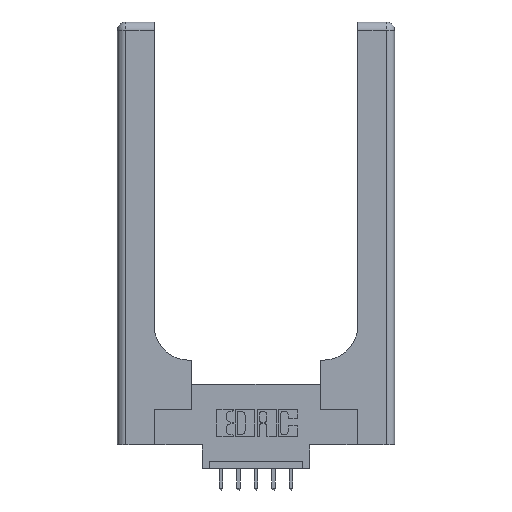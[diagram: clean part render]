
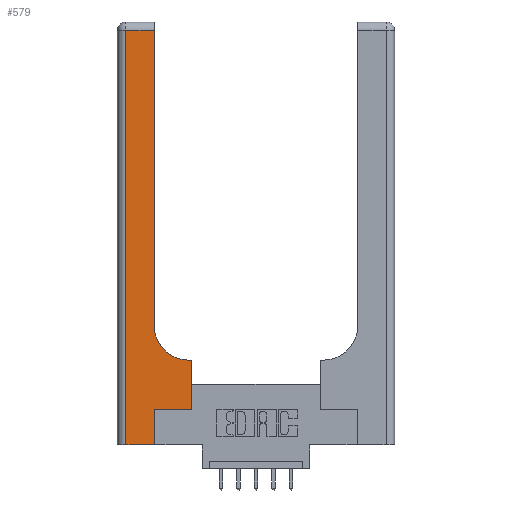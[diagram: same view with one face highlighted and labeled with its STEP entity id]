
A CAD part, top view. The second image highlights one B-rep face of the part: STEP entity #579.
In plain terms, the highlighted planar face has unit normal (0, 0, 1).
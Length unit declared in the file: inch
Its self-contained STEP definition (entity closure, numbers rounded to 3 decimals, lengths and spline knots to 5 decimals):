
#251 = VECTOR ( 'NONE', #9648, 39.37008 ) ;
#280 = VERTEX_POINT ( 'NONE', #6161 ) ;
#362 = CARTESIAN_POINT ( 'NONE',  ( 0.528, 0.25, 0.37 ) ) ;
#579 = ADVANCED_FACE ( 'NONE', ( #1124 ), #13851, .F. ) ;
#590 = DIRECTION ( 'NONE',  ( -1., 0., 0. ) ) ;
#598 = EDGE_CURVE ( 'NONE', #6962, #11774, #5293, .T. ) ;
#700 = AXIS2_PLACEMENT_3D ( 'NONE', #12774, #4372, #6391 ) ;
#1124 = FACE_OUTER_BOUND ( 'NONE', #13270, .T. ) ;
#1232 = DIRECTION ( 'NONE',  ( 0., 1., 0. ) ) ;
#1258 = EDGE_CURVE ( 'NONE', #1387, #6962, #11428, .T. ) ;
#1387 = VERTEX_POINT ( 'NONE', #4468 ) ;
#1480 = CARTESIAN_POINT ( 'NONE',  ( 0.26, 0.85, 0.37 ) ) ;
#1696 = CARTESIAN_POINT ( 'NONE',  ( 0.265, 0., 0.37 ) ) ;
#1925 = CARTESIAN_POINT ( 'NONE',  ( 0.06, 3., 0.37 ) ) ;
#2187 = ORIENTED_EDGE ( 'NONE', *, *, #9672, .T. ) ;
#2524 = CARTESIAN_POINT ( 'NONE',  ( 0.528, 0.6, 0.37 ) ) ;
#2582 = ORIENTED_EDGE ( 'NONE', *, *, #7468, .T. ) ;
#2617 = DIRECTION ( 'NONE',  ( 1., 0., 0. ) ) ;
#3058 = LINE ( 'NONE', #7111, #8286 ) ;
#3175 = AXIS2_PLACEMENT_3D ( 'NONE', #3358, #4491, #8516 ) ;
#3358 = CARTESIAN_POINT ( 'NONE',  ( 0., 3., 0.37 ) ) ;
#3523 = CARTESIAN_POINT ( 'NONE',  ( 0., 0., 0.37 ) ) ;
#4240 = CARTESIAN_POINT ( 'NONE',  ( 0.06, 2.94, 0.37 ) ) ;
#4372 = DIRECTION ( 'NONE',  ( 0., 0., -1. ) ) ;
#4468 = CARTESIAN_POINT ( 'NONE',  ( 0.51, 0.6, 0.37 ) ) ;
#4491 = DIRECTION ( 'NONE',  ( 0., 0., -1. ) ) ;
#4892 = VECTOR ( 'NONE', #6206, 39.37008 ) ;
#4983 = EDGE_CURVE ( 'NONE', #280, #12403, #9794, .T. ) ;
#5293 = LINE ( 'NONE', #9505, #251 ) ;
#5729 = ORIENTED_EDGE ( 'NONE', *, *, #4983, .T. ) ;
#5909 = LINE ( 'NONE', #7218, #11652 ) ;
#5926 = LINE ( 'NONE', #6195, #9337 ) ;
#5985 = DIRECTION ( 'NONE',  ( 0., 1., 0. ) ) ;
#6002 = DIRECTION ( 'NONE',  ( 1., 0., 0. ) ) ;
#6140 = VECTOR ( 'NONE', #11436, 39.37008 ) ;
#6161 = CARTESIAN_POINT ( 'NONE',  ( 0.528, 0.25, 0.37 ) ) ;
#6195 = CARTESIAN_POINT ( 'NONE',  ( 0.265, 0.25, 0.37 ) ) ;
#6206 = DIRECTION ( 'NONE',  ( 0., -1., 0. ) ) ;
#6214 = CARTESIAN_POINT ( 'NONE',  ( 0.265, 0.25, 0.37 ) ) ;
#6215 = LINE ( 'NONE', #7385, #6140 ) ;
#6391 = DIRECTION ( 'NONE',  ( 1., 0., 0. ) ) ;
#6962 = VERTEX_POINT ( 'NONE', #1480 ) ;
#6969 = ORIENTED_EDGE ( 'NONE', *, *, #598, .T. ) ;
#7111 = CARTESIAN_POINT ( 'NONE',  ( 0., 2.94, 0.37 ) ) ;
#7218 = CARTESIAN_POINT ( 'NONE',  ( 0.265, 0., 0.37 ) ) ;
#7385 = CARTESIAN_POINT ( 'NONE',  ( 0.26, 0.6, 0.37 ) ) ;
#7468 = EDGE_CURVE ( 'NONE', #12069, #8774, #11512, .T. ) ;
#7516 = ORIENTED_EDGE ( 'NONE', *, *, #12273, .T. ) ;
#8286 = VECTOR ( 'NONE', #590, 39.37008 ) ;
#8392 = LINE ( 'NONE', #3523, #11924 ) ;
#8516 = DIRECTION ( 'NONE',  ( -1., 0., 0. ) ) ;
#8590 = VECTOR ( 'NONE', #1232, 39.37008 ) ;
#8774 = VERTEX_POINT ( 'NONE', #10991 ) ;
#8903 = ORIENTED_EDGE ( 'NONE', *, *, #1258, .T. ) ;
#9337 = VECTOR ( 'NONE', #6002, 39.37008 ) ;
#9494 = EDGE_CURVE ( 'NONE', #11774, #12069, #3058, .T. ) ;
#9505 = CARTESIAN_POINT ( 'NONE',  ( 0.26, 3., 0.37 ) ) ;
#9648 = DIRECTION ( 'NONE',  ( 0., 1., 0. ) ) ;
#9672 = EDGE_CURVE ( 'NONE', #9706, #12047, #5909, .T. ) ;
#9706 = VERTEX_POINT ( 'NONE', #1696 ) ;
#9794 = LINE ( 'NONE', #362, #8590 ) ;
#9906 = ORIENTED_EDGE ( 'NONE', *, *, #10032, .T. ) ;
#10032 = EDGE_CURVE ( 'NONE', #12047, #280, #5926, .T. ) ;
#10991 = CARTESIAN_POINT ( 'NONE',  ( 0.06, 0., 0.37 ) ) ;
#11428 = CIRCLE ( 'NONE', #700, 0.25 ) ;
#11436 = DIRECTION ( 'NONE',  ( -1., 0., 0. ) ) ;
#11512 = LINE ( 'NONE', #1925, #4892 ) ;
#11652 = VECTOR ( 'NONE', #5985, 39.37008 ) ;
#11699 = ORIENTED_EDGE ( 'NONE', *, *, #12658, .T. ) ;
#11774 = VERTEX_POINT ( 'NONE', #13467 ) ;
#11924 = VECTOR ( 'NONE', #2617, 39.37008 ) ;
#12047 = VERTEX_POINT ( 'NONE', #6214 ) ;
#12069 = VERTEX_POINT ( 'NONE', #4240 ) ;
#12273 = EDGE_CURVE ( 'NONE', #8774, #9706, #8392, .T. ) ;
#12403 = VERTEX_POINT ( 'NONE', #2524 ) ;
#12658 = EDGE_CURVE ( 'NONE', #12403, #1387, #6215, .T. ) ;
#12774 = CARTESIAN_POINT ( 'NONE',  ( 0.51, 0.85, 0.37 ) ) ;
#12940 = ORIENTED_EDGE ( 'NONE', *, *, #9494, .T. ) ;
#13270 = EDGE_LOOP ( 'NONE', ( #6969, #12940, #2582, #7516, #2187, #9906, #5729, #11699, #8903 ) ) ;
#13467 = CARTESIAN_POINT ( 'NONE',  ( 0.26, 2.94, 0.37 ) ) ;
#13851 = PLANE ( 'NONE',  #3175 ) ;
